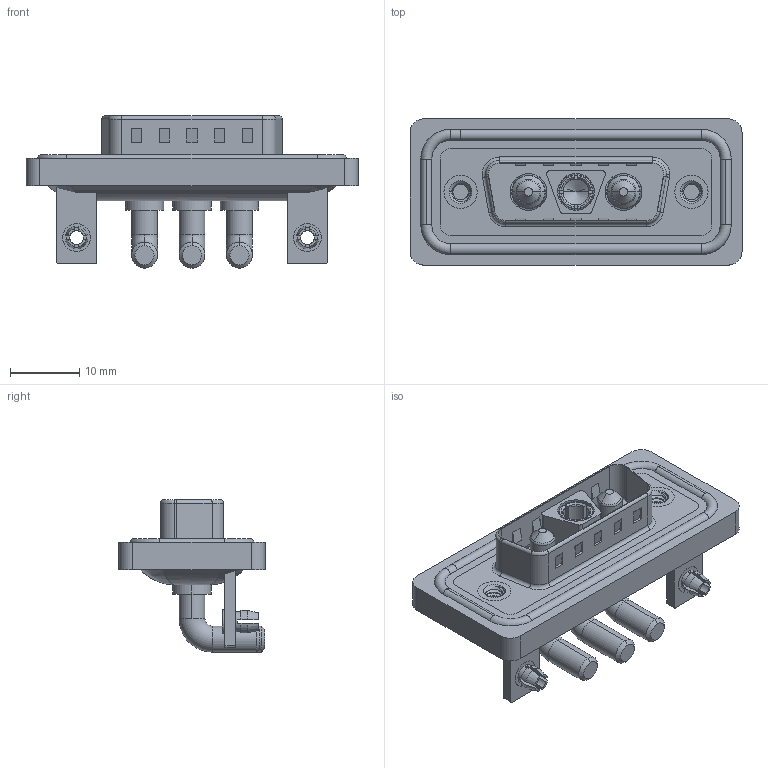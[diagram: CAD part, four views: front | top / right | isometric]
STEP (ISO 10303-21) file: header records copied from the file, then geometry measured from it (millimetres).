
FILE_DESCRIPTION (( 'STEP AP203' ), '1' );
FILE_NAME ('629W3WK3140-4N3.STEP', '2024-04-11T13:32:12', ( '' ), ( '' ), 'SwSTEP 2.0', 'SolidWorks 2023', '' );
FILE_SCHEMA (( 'CONFIG_CONTROL_DESIGN' ));
Length unit declared in the file: millimetre
Products named in the file (10): 629Combo Housing_3WK3; 629W3WK3140-4N3; 629Combo Shell Rear_15 Contacts; 629Combo Board Lock; 629Combo Threaded Rivet_3; Power Pin_40A RA; 629Combo Shell Front_15 Contacts; Power Socket_40A RA; 629Combo Stabilizer Bracket; 629Combo Waterproof Housing_15 Contacts
Assembly tree (13 placements, depth 2):
  629W3WK3140-4N3
    629Combo Housing_3WK3
    629Combo Shell Rear_15 Contacts
    629Combo Shell Front_15 Contacts
    629Combo Waterproof Housing_15 Contacts
    629Combo Threaded Rivet_3  x2
    629Combo Stabilizer Bracket  x2
    629Combo Board Lock  x2
    Power Socket_40A RA
    Power Pin_40A RA  x2
Bounding box: 47.9 x 21.1 x 21.98 mm (x, y, z)
Volume: 6421 mm3; surface area: 10346.9 mm2
Topology: 17 solids, 17 shells, 753 faces, 1896 edges, 1202 vertices
Faces by surface type: cylinder 306, plane 299, torus 78, cone 57, bspline 13
Entity records: 21638 total; most frequent: CARTESIAN_POINT 5295, DIRECTION 3320, ORIENTED_EDGE 3100, EDGE_CURVE 1550, AXIS2_PLACEMENT_3D 1256, VERTEX_POINT 987, VECTOR 808, LINE 808
